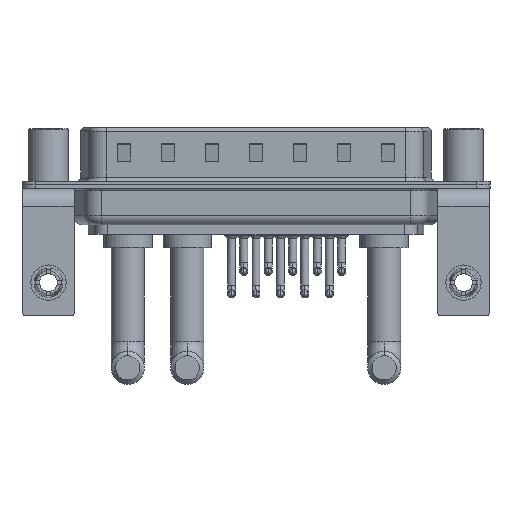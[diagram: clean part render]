
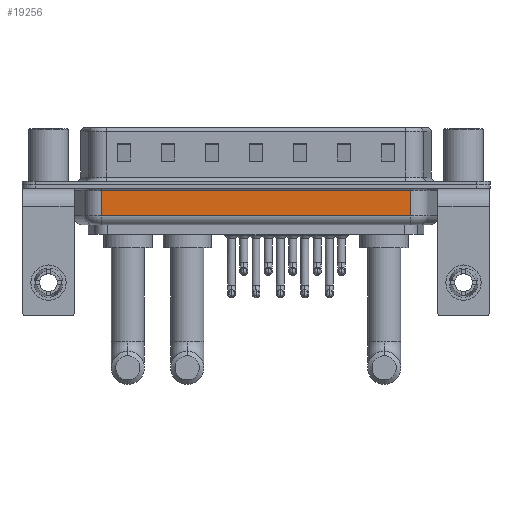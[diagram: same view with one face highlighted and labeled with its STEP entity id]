
A CAD part, front view. The second image highlights one B-rep face of the part: STEP entity #19256.
In plain terms, the highlighted planar face has unit normal (0, -1, 0).
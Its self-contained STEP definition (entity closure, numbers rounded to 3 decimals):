
#327 = ORIENTED_EDGE ( 'NONE', *, *, #19908, .F. ) ;
#1633 = VERTEX_POINT ( 'NONE', #7221 ) ;
#3984 = VERTEX_POINT ( 'NONE', #17040 ) ;
#4858 = CARTESIAN_POINT ( 'NONE',  ( 6.006, -5.35, -4.5 ) ) ;
#6021 = VERTEX_POINT ( 'NONE', #26915 ) ;
#6049 = LINE ( 'NONE', #10159, #19676 ) ;
#7052 = DIRECTION ( 'NONE',  ( 0., 0., 1. ) ) ;
#7221 = CARTESIAN_POINT ( 'NONE',  ( 41.044, -5.35, -0.65 ) ) ;
#8454 = ORIENTED_EDGE ( 'NONE', *, *, #22118, .T. ) ;
#8967 = FACE_OUTER_BOUND ( 'NONE', #18589, .T. ) ;
#9234 = LINE ( 'NONE', #23511, #9398 ) ;
#9398 = VECTOR ( 'NONE', #22877, 1000. ) ;
#10159 = CARTESIAN_POINT ( 'NONE',  ( 6.006, -5.35, -4.5 ) ) ;
#11584 = ORIENTED_EDGE ( 'NONE', *, *, #17936, .T. ) ;
#12609 = AXIS2_PLACEMENT_3D ( 'NONE', #4858, #19696, #7052 ) ;
#13782 = EDGE_CURVE ( 'NONE', #1633, #14708, #9234, .T. ) ;
#14358 = ORIENTED_EDGE ( 'NONE', *, *, #13782, .T. ) ;
#14554 = DIRECTION ( 'NONE',  ( 0., 0., 1. ) ) ;
#14587 = DIRECTION ( 'NONE',  ( 1., 0., 0. ) ) ;
#14708 = VERTEX_POINT ( 'NONE', #15175 ) ;
#15175 = CARTESIAN_POINT ( 'NONE',  ( 6.006, -5.35, -0.65 ) ) ;
#15297 = PLANE ( 'NONE',  #12609 ) ;
#16508 = VECTOR ( 'NONE', #17334, 1000. ) ;
#16510 = CARTESIAN_POINT ( 'NONE',  ( 6.006, -5.35, -3.5 ) ) ;
#16764 = LINE ( 'NONE', #16510, #19339 ) ;
#17040 = CARTESIAN_POINT ( 'NONE',  ( 41.044, -5.35, -3.5 ) ) ;
#17334 = DIRECTION ( 'NONE',  ( 0., 0., 1. ) ) ;
#17936 = EDGE_CURVE ( 'NONE', #3984, #1633, #25984, .T. ) ;
#18589 = EDGE_LOOP ( 'NONE', ( #327, #8454, #11584, #14358 ) ) ;
#19256 = ADVANCED_FACE ( 'NONE', ( #8967 ), #15297, .F. ) ;
#19339 = VECTOR ( 'NONE', #14587, 1000. ) ;
#19676 = VECTOR ( 'NONE', #14554, 1000. ) ;
#19696 = DIRECTION ( 'NONE',  ( 0., 1., 0. ) ) ;
#19908 = EDGE_CURVE ( 'NONE', #6021, #14708, #6049, .T. ) ;
#21744 = CARTESIAN_POINT ( 'NONE',  ( 41.044, -5.35, -4.5 ) ) ;
#22118 = EDGE_CURVE ( 'NONE', #6021, #3984, #16764, .T. ) ;
#22877 = DIRECTION ( 'NONE',  ( -1., 0., 0. ) ) ;
#23511 = CARTESIAN_POINT ( 'NONE',  ( 6.006, -5.35, -0.65 ) ) ;
#25984 = LINE ( 'NONE', #21744, #16508 ) ;
#26915 = CARTESIAN_POINT ( 'NONE',  ( 6.006, -5.35, -3.5 ) ) ;
